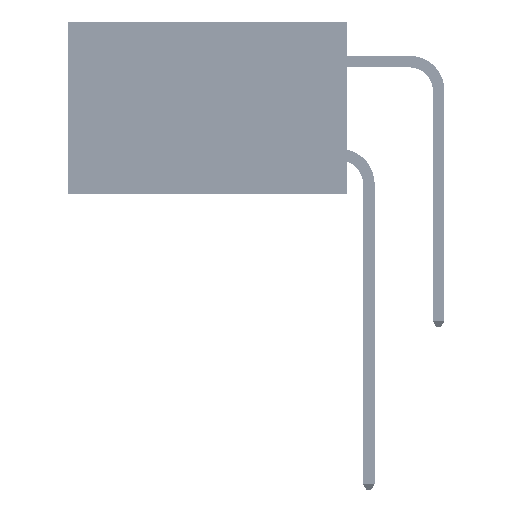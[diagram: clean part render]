
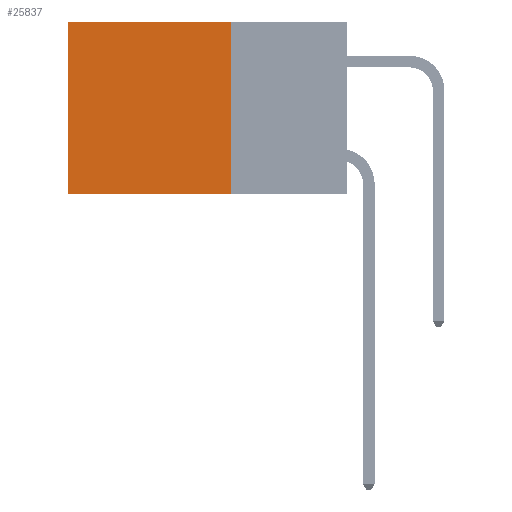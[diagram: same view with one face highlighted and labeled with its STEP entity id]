
A CAD part, left-side view. The second image highlights one B-rep face of the part: STEP entity #25837.
In plain terms, the highlighted planar face has unit normal (-1, 0, 0).
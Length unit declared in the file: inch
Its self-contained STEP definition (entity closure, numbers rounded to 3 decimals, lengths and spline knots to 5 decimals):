
#175 = DIRECTION ( 'NONE',  ( 0., 0., -1. ) ) ;
#1514 = CARTESIAN_POINT ( 'NONE',  ( 0.2875, 0.6, -0.37 ) ) ;
#3354 = LINE ( 'NONE', #4156, #51312 ) ;
#4156 = CARTESIAN_POINT ( 'NONE',  ( 0.2875, 0.25, -0.37 ) ) ;
#5509 = DIRECTION ( 'NONE',  ( 0., 0., -1. ) ) ;
#5802 = CARTESIAN_POINT ( 'NONE',  ( 0.2875, 0.25, 0. ) ) ;
#6807 = EDGE_CURVE ( 'NONE', #28259, #27005, #39070, .T. ) ;
#8371 = VECTOR ( 'NONE', #10851, 39.37008 ) ;
#8439 = VECTOR ( 'NONE', #5509, 39.37008 ) ;
#9599 = EDGE_CURVE ( 'NONE', #27005, #42649, #35432, .T. ) ;
#10851 = DIRECTION ( 'NONE',  ( 0., 1., 0. ) ) ;
#11226 = CARTESIAN_POINT ( 'NONE',  ( 0.2875, 0.25, 0. ) ) ;
#11907 = FACE_OUTER_BOUND ( 'NONE', #26581, .T. ) ;
#12176 = ORIENTED_EDGE ( 'NONE', *, *, #9599, .T. ) ;
#14667 = CARTESIAN_POINT ( 'NONE',  ( 0.2875, 0.6, 0. ) ) ;
#14834 = CARTESIAN_POINT ( 'NONE',  ( 0.2875, 0.25, 0. ) ) ;
#15363 = CARTESIAN_POINT ( 'NONE',  ( 0.2875, 0.6, 0. ) ) ;
#18932 = DIRECTION ( 'NONE',  ( 0., 0., -1. ) ) ;
#19813 = EDGE_CURVE ( 'NONE', #47003, #42649, #3354, .T. ) ;
#20394 = DIRECTION ( 'NONE',  ( 0., 1., 0. ) ) ;
#20559 = VECTOR ( 'NONE', #18932, 39.37008 ) ;
#20665 = DIRECTION ( 'NONE',  ( 1., 0., 0. ) ) ;
#24090 = ORIENTED_EDGE ( 'NONE', *, *, #39402, .F. ) ;
#25201 = AXIS2_PLACEMENT_3D ( 'NONE', #40399, #20665, #175 ) ;
#25837 = ADVANCED_FACE ( 'NONE', ( #11907 ), #36654, .F. ) ;
#26581 = EDGE_LOOP ( 'NONE', ( #12176, #46205, #24090, #33727 ) ) ;
#27005 = VERTEX_POINT ( 'NONE', #15363 ) ;
#28259 = VERTEX_POINT ( 'NONE', #14834 ) ;
#33727 = ORIENTED_EDGE ( 'NONE', *, *, #6807, .T. ) ;
#35432 = LINE ( 'NONE', #14667, #8439 ) ;
#36415 = CARTESIAN_POINT ( 'NONE',  ( 0.2875, 0.25, -0.37 ) ) ;
#36654 = PLANE ( 'NONE',  #25201 ) ;
#39070 = LINE ( 'NONE', #5802, #8371 ) ;
#39402 = EDGE_CURVE ( 'NONE', #28259, #47003, #43158, .T. ) ;
#40399 = CARTESIAN_POINT ( 'NONE',  ( 0.2875, 0.25, 0. ) ) ;
#42649 = VERTEX_POINT ( 'NONE', #1514 ) ;
#43158 = LINE ( 'NONE', #11226, #20559 ) ;
#46205 = ORIENTED_EDGE ( 'NONE', *, *, #19813, .F. ) ;
#47003 = VERTEX_POINT ( 'NONE', #36415 ) ;
#51312 = VECTOR ( 'NONE', #20394, 39.37008 ) ;
